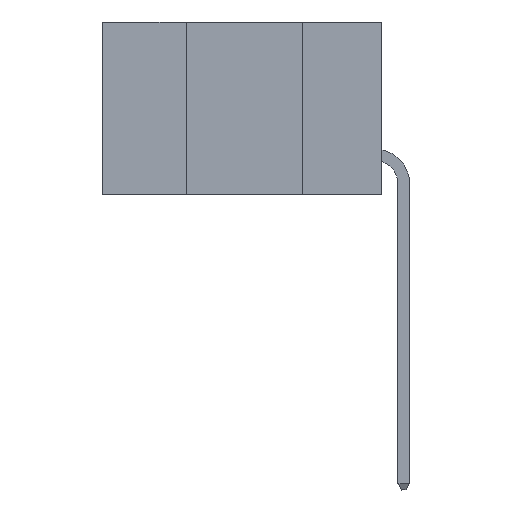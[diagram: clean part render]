
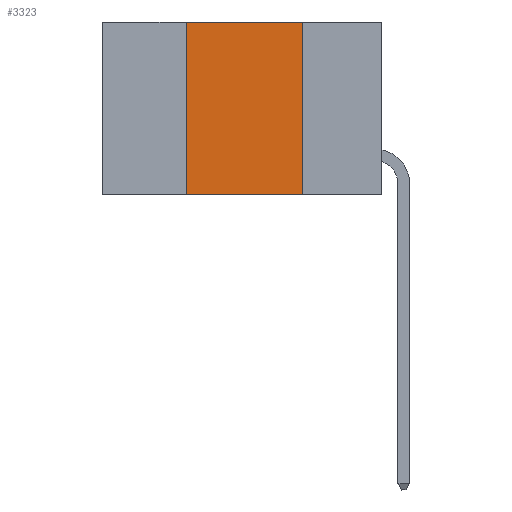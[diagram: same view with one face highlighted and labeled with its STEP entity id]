
A CAD part, left-side view. The second image highlights one B-rep face of the part: STEP entity #3323.
In plain terms, the highlighted planar face has unit normal (-1, 0, 0).
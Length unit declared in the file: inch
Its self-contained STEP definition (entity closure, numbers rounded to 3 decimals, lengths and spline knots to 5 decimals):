
#692 = LINE ( 'NONE', #16844, #2385 ) ;
#1196 = VERTEX_POINT ( 'NONE', #17903 ) ;
#1215 = EDGE_CURVE ( 'NONE', #1196, #21028, #3040, .T. ) ;
#2385 = VECTOR ( 'NONE', #6000, 39.37008 ) ;
#3040 = LINE ( 'NONE', #23346, #22234 ) ;
#3323 = ADVANCED_FACE ( 'NONE', ( #25773 ), #4673, .F. ) ;
#4224 = ORIENTED_EDGE ( 'NONE', *, *, #1215, .F. ) ;
#4673 = PLANE ( 'NONE',  #26543 ) ;
#4883 = DIRECTION ( 'NONE',  ( 0., 0., -1. ) ) ;
#6000 = DIRECTION ( 'NONE',  ( 0., -1., 0. ) ) ;
#8255 = ORIENTED_EDGE ( 'NONE', *, *, #8750, .F. ) ;
#8750 = EDGE_CURVE ( 'NONE', #9600, #14072, #22561, .T. ) ;
#9600 = VERTEX_POINT ( 'NONE', #25091 ) ;
#10032 = DIRECTION ( 'NONE',  ( 1., 0., 0. ) ) ;
#10068 = DIRECTION ( 'NONE',  ( 0., -1., 0. ) ) ;
#12886 = EDGE_CURVE ( 'NONE', #1196, #14072, #24657, .T. ) ;
#14072 = VERTEX_POINT ( 'NONE', #26751 ) ;
#15200 = VECTOR ( 'NONE', #10068, 39.37008 ) ;
#16478 = DIRECTION ( 'NONE',  ( 0., 0., -1. ) ) ;
#16844 = CARTESIAN_POINT ( 'NONE',  ( 0., 0.6, 0. ) ) ;
#17903 = CARTESIAN_POINT ( 'NONE',  ( 0., 0.42, -0.37 ) ) ;
#17924 = CARTESIAN_POINT ( 'NONE',  ( 0., 0.6, -0.37 ) ) ;
#18113 = CARTESIAN_POINT ( 'NONE',  ( 0., 0.6, 0. ) ) ;
#20143 = ORIENTED_EDGE ( 'NONE', *, *, #27957, .F. ) ;
#21028 = VERTEX_POINT ( 'NONE', #29475 ) ;
#22234 = VECTOR ( 'NONE', #23231, 39.37008 ) ;
#22561 = LINE ( 'NONE', #26571, #23372 ) ;
#23231 = DIRECTION ( 'NONE',  ( 0., 0., 1. ) ) ;
#23346 = CARTESIAN_POINT ( 'NONE',  ( 0., 0.42, 0. ) ) ;
#23372 = VECTOR ( 'NONE', #16478, 39.37008 ) ;
#24657 = LINE ( 'NONE', #17924, #15200 ) ;
#25091 = CARTESIAN_POINT ( 'NONE',  ( 0., 0.17, 0. ) ) ;
#25725 = ORIENTED_EDGE ( 'NONE', *, *, #12886, .T. ) ;
#25773 = FACE_OUTER_BOUND ( 'NONE', #28969, .T. ) ;
#26543 = AXIS2_PLACEMENT_3D ( 'NONE', #18113, #10032, #4883 ) ;
#26571 = CARTESIAN_POINT ( 'NONE',  ( 0., 0.17, 0. ) ) ;
#26751 = CARTESIAN_POINT ( 'NONE',  ( 0., 0.17, -0.37 ) ) ;
#27957 = EDGE_CURVE ( 'NONE', #21028, #9600, #692, .T. ) ;
#28969 = EDGE_LOOP ( 'NONE', ( #8255, #20143, #4224, #25725 ) ) ;
#29475 = CARTESIAN_POINT ( 'NONE',  ( 0., 0.42, 0. ) ) ;
